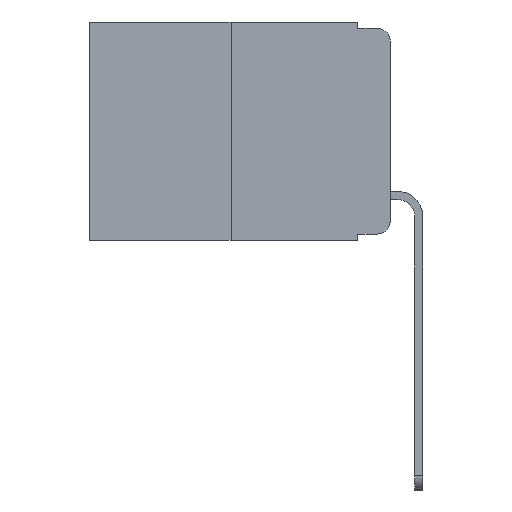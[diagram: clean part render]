
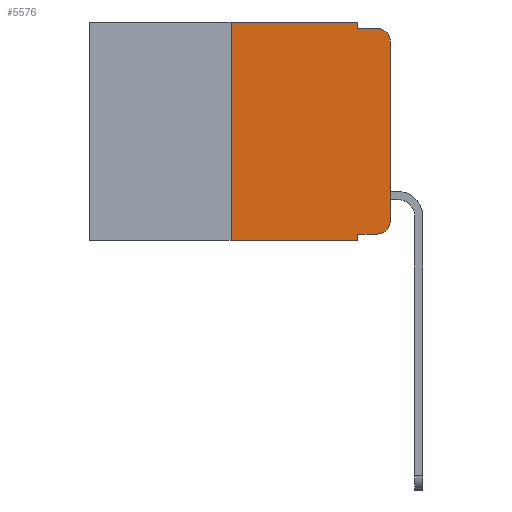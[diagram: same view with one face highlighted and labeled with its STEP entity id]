
A CAD part, left-side view. The second image highlights one B-rep face of the part: STEP entity #5576.
In plain terms, the highlighted planar face has unit normal (-1, 0, 0).
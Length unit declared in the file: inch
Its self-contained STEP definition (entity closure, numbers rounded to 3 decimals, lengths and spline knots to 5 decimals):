
#598 = PLANE ( 'NONE',  #20090 ) ;
#740 = VERTEX_POINT ( 'NONE', #13889 ) ;
#1034 = VECTOR ( 'NONE', #18749, 39.37008 ) ;
#1363 = ORIENTED_EDGE ( 'NONE', *, *, #3761, .F. ) ;
#1547 = LINE ( 'NONE', #10906, #1034 ) ;
#1557 = ORIENTED_EDGE ( 'NONE', *, *, #13573, .F. ) ;
#1678 = VECTOR ( 'NONE', #12410, 39.37008 ) ;
#2546 = CARTESIAN_POINT ( 'NONE',  ( 0., 0.473, -0.343 ) ) ;
#2719 = VECTOR ( 'NONE', #7795, 39.37008 ) ;
#2823 = CARTESIAN_POINT ( 'NONE',  ( 0., 0., -0.313 ) ) ;
#3041 = EDGE_CURVE ( 'NONE', #3398, #17043, #8940, .T. ) ;
#3398 = VERTEX_POINT ( 'NONE', #7872 ) ;
#3507 = VERTEX_POINT ( 'NONE', #10365 ) ;
#3579 = AXIS2_PLACEMENT_3D ( 'NONE', #11211, #15960, #6579 ) ;
#3618 = EDGE_CURVE ( 'NONE', #14322, #10098, #10531, .T. ) ;
#3761 = EDGE_CURVE ( 'NONE', #3507, #18574, #8591, .T. ) ;
#3780 = LINE ( 'NONE', #14436, #15348 ) ;
#4317 = EDGE_CURVE ( 'NONE', #10138, #12296, #15165, .T. ) ;
#4393 = VECTOR ( 'NONE', #17642, 39.37008 ) ;
#4458 = ORIENTED_EDGE ( 'NONE', *, *, #3041, .F. ) ;
#4564 = DIRECTION ( 'NONE',  ( 0., 0., -1. ) ) ;
#5576 = ADVANCED_FACE ( 'NONE', ( #19784 ), #598, .F. ) ;
#6139 = EDGE_CURVE ( 'NONE', #18574, #740, #1547, .T. ) ;
#6579 = DIRECTION ( 'NONE',  ( 0., 0., -1. ) ) ;
#6705 = DIRECTION ( 'NONE',  ( 0., -1., 0. ) ) ;
#6818 = EDGE_LOOP ( 'NONE', ( #19891, #9458, #7621, #1363, #1557, #4458, #9148, #18675, #8354, #19282 ) ) ;
#7043 = DIRECTION ( 'NONE',  ( 0., 0., -1. ) ) ;
#7166 = AXIS2_PLACEMENT_3D ( 'NONE', #15464, #13942, #4564 ) ;
#7252 = VERTEX_POINT ( 'NONE', #17698 ) ;
#7621 = ORIENTED_EDGE ( 'NONE', *, *, #6139, .F. ) ;
#7795 = DIRECTION ( 'NONE',  ( 0., 0., 1. ) ) ;
#7872 = CARTESIAN_POINT ( 'NONE',  ( 0., 0.25, -0.343 ) ) ;
#7898 = DIRECTION ( 'NONE',  ( 0., 0., 1. ) ) ;
#8349 = VECTOR ( 'NONE', #14080, 39.37008 ) ;
#8354 = ORIENTED_EDGE ( 'NONE', *, *, #19207, .T. ) ;
#8591 = LINE ( 'NONE', #15728, #8349 ) ;
#8644 = CIRCLE ( 'NONE', #7166, 0.02 ) ;
#8940 = LINE ( 'NONE', #15514, #2719 ) ;
#9148 = ORIENTED_EDGE ( 'NONE', *, *, #16125, .T. ) ;
#9197 = CARTESIAN_POINT ( 'NONE',  ( 0., 0.051, -0.333 ) ) ;
#9458 = ORIENTED_EDGE ( 'NONE', *, *, #16935, .T. ) ;
#9540 = CARTESIAN_POINT ( 'NONE',  ( 0., 0., 0. ) ) ;
#9554 = CARTESIAN_POINT ( 'NONE',  ( 0., 0.051, -0.01 ) ) ;
#10098 = VERTEX_POINT ( 'NONE', #10716 ) ;
#10138 = VERTEX_POINT ( 'NONE', #2823 ) ;
#10365 = CARTESIAN_POINT ( 'NONE',  ( 0., 0.051, 0. ) ) ;
#10531 = LINE ( 'NONE', #19281, #4393 ) ;
#10716 = CARTESIAN_POINT ( 'NONE',  ( 0., 0.051, -0.343 ) ) ;
#10906 = CARTESIAN_POINT ( 'NONE',  ( 0., 0.051, -0.01 ) ) ;
#11211 = CARTESIAN_POINT ( 'NONE',  ( 0., 0.02, -0.313 ) ) ;
#11590 = CARTESIAN_POINT ( 'NONE',  ( 0., 0.473, 0. ) ) ;
#12296 = VERTEX_POINT ( 'NONE', #12390 ) ;
#12390 = CARTESIAN_POINT ( 'NONE',  ( 0., 0., -0.03 ) ) ;
#12410 = DIRECTION ( 'NONE',  ( 0., -1., 0. ) ) ;
#13573 = EDGE_CURVE ( 'NONE', #17043, #3507, #17720, .T. ) ;
#13662 = VECTOR ( 'NONE', #7898, 39.37008 ) ;
#13889 = CARTESIAN_POINT ( 'NONE',  ( 0., 0.02, -0.01 ) ) ;
#13942 = DIRECTION ( 'NONE',  ( -1., 0., 0. ) ) ;
#14027 = CIRCLE ( 'NONE', #3579, 0.02 ) ;
#14080 = DIRECTION ( 'NONE',  ( 0., 0., -1. ) ) ;
#14322 = VERTEX_POINT ( 'NONE', #9197 ) ;
#14436 = CARTESIAN_POINT ( 'NONE',  ( 0., 0.051, -0.333 ) ) ;
#15056 = VECTOR ( 'NONE', #19764, 39.37008 ) ;
#15165 = LINE ( 'NONE', #9540, #13662 ) ;
#15348 = VECTOR ( 'NONE', #6705, 39.37008 ) ;
#15464 = CARTESIAN_POINT ( 'NONE',  ( 0., 0.02, -0.03 ) ) ;
#15514 = CARTESIAN_POINT ( 'NONE',  ( 0., 0.25, 0. ) ) ;
#15728 = CARTESIAN_POINT ( 'NONE',  ( 0., 0.051, 0. ) ) ;
#15960 = DIRECTION ( 'NONE',  ( -1., 0., 0. ) ) ;
#16125 = EDGE_CURVE ( 'NONE', #3398, #10098, #19731, .T. ) ;
#16419 = DIRECTION ( 'NONE',  ( 1., 0., 0. ) ) ;
#16736 = EDGE_CURVE ( 'NONE', #7252, #10138, #14027, .T. ) ;
#16935 = EDGE_CURVE ( 'NONE', #12296, #740, #8644, .T. ) ;
#17043 = VERTEX_POINT ( 'NONE', #17274 ) ;
#17274 = CARTESIAN_POINT ( 'NONE',  ( 0., 0.25, 0. ) ) ;
#17642 = DIRECTION ( 'NONE',  ( 0., 0., -1. ) ) ;
#17698 = CARTESIAN_POINT ( 'NONE',  ( 0., 0.02, -0.333 ) ) ;
#17720 = LINE ( 'NONE', #18849, #1678 ) ;
#18574 = VERTEX_POINT ( 'NONE', #9554 ) ;
#18675 = ORIENTED_EDGE ( 'NONE', *, *, #3618, .F. ) ;
#18749 = DIRECTION ( 'NONE',  ( 0., -1., 0. ) ) ;
#18849 = CARTESIAN_POINT ( 'NONE',  ( 0., 0.473, 0. ) ) ;
#19207 = EDGE_CURVE ( 'NONE', #14322, #7252, #3780, .T. ) ;
#19281 = CARTESIAN_POINT ( 'NONE',  ( 0., 0.051, 0. ) ) ;
#19282 = ORIENTED_EDGE ( 'NONE', *, *, #16736, .T. ) ;
#19731 = LINE ( 'NONE', #2546, #15056 ) ;
#19764 = DIRECTION ( 'NONE',  ( 0., -1., 0. ) ) ;
#19784 = FACE_OUTER_BOUND ( 'NONE', #6818, .T. ) ;
#19891 = ORIENTED_EDGE ( 'NONE', *, *, #4317, .T. ) ;
#20090 = AXIS2_PLACEMENT_3D ( 'NONE', #11590, #16419, #7043 ) ;
